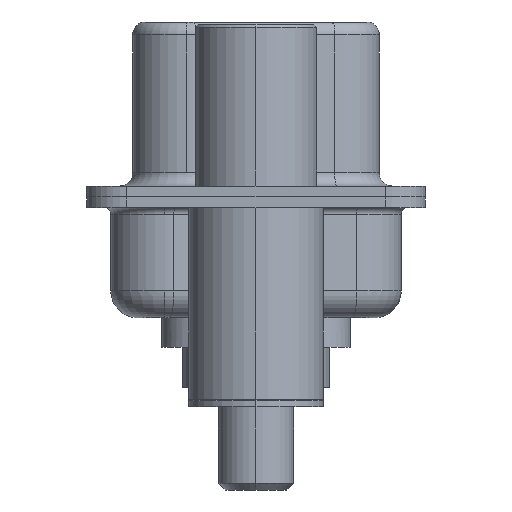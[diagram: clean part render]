
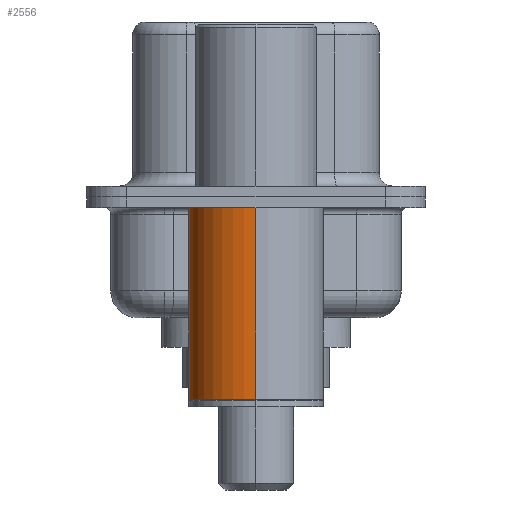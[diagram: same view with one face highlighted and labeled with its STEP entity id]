
A CAD part, left-side view. The second image highlights one B-rep face of the part: STEP entity #2556.
In plain terms, the highlighted cylindrical face has radius 2.5 mm (diameter 5 mm), a partial arc.
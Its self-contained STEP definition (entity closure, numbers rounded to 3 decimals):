
#69 = ORIENTED_EDGE ( 'NONE', *, *, #9008, .F. ) ;
#408 = CARTESIAN_POINT ( 'NONE',  ( -2.5, 0., -0.4 ) ) ;
#678 = DIRECTION ( 'NONE',  ( 0., 0., 1. ) ) ;
#1037 = DIRECTION ( 'NONE',  ( 0., 0., 1. ) ) ;
#2556 = ADVANCED_FACE ( 'NONE', ( #15128 ), #6331, .T. ) ;
#2654 = VERTEX_POINT ( 'NONE', #3700 ) ;
#2798 = CARTESIAN_POINT ( 'NONE',  ( 0., 0., 0.581 ) ) ;
#3330 = CARTESIAN_POINT ( 'NONE',  ( 2.5, 0., 0.581 ) ) ;
#3400 = DIRECTION ( 'NONE',  ( 0., 0., 1. ) ) ;
#3700 = CARTESIAN_POINT ( 'NONE',  ( 2.5, 0., -0.4 ) ) ;
#5219 = CIRCLE ( 'NONE', #7861, 2.5 ) ;
#5476 = ORIENTED_EDGE ( 'NONE', *, *, #16485, .T. ) ;
#6331 = CYLINDRICAL_SURFACE ( 'NONE', #12950, 2.5 ) ;
#6455 = CARTESIAN_POINT ( 'NONE',  ( 0., 0., -7.525 ) ) ;
#7040 = AXIS2_PLACEMENT_3D ( 'NONE', #6455, #18006, #8164 ) ;
#7615 = VERTEX_POINT ( 'NONE', #17468 ) ;
#7847 = LINE ( 'NONE', #3330, #16074 ) ;
#7861 = AXIS2_PLACEMENT_3D ( 'NONE', #10908, #1037, #12555 ) ;
#8020 = EDGE_LOOP ( 'NONE', ( #13777, #5476, #69, #21272 ) ) ;
#8109 = VERTEX_POINT ( 'NONE', #408 ) ;
#8164 = DIRECTION ( 'NONE',  ( 1., 0., 0. ) ) ;
#8531 = VECTOR ( 'NONE', #8851, 1000. ) ;
#8851 = DIRECTION ( 'NONE',  ( 0., 0., 1. ) ) ;
#9008 = EDGE_CURVE ( 'NONE', #2654, #8109, #5219, .T. ) ;
#10472 = VERTEX_POINT ( 'NONE', #19697 ) ;
#10908 = CARTESIAN_POINT ( 'NONE',  ( 0., 0., -0.4 ) ) ;
#11672 = EDGE_CURVE ( 'NONE', #10472, #7615, #12080, .T. ) ;
#12080 = CIRCLE ( 'NONE', #7040, 2.5 ) ;
#12555 = DIRECTION ( 'NONE',  ( 1., 0., 0. ) ) ;
#12835 = LINE ( 'NONE', #15351, #8531 ) ;
#12950 = AXIS2_PLACEMENT_3D ( 'NONE', #2798, #678, #20352 ) ;
#13777 = ORIENTED_EDGE ( 'NONE', *, *, #11672, .T. ) ;
#15128 = FACE_OUTER_BOUND ( 'NONE', #8020, .T. ) ;
#15351 = CARTESIAN_POINT ( 'NONE',  ( -2.5, 0., 0.581 ) ) ;
#16074 = VECTOR ( 'NONE', #3400, 1000. ) ;
#16485 = EDGE_CURVE ( 'NONE', #7615, #8109, #12835, .T. ) ;
#17468 = CARTESIAN_POINT ( 'NONE',  ( -2.5, 0., -7.525 ) ) ;
#18006 = DIRECTION ( 'NONE',  ( 0., 0., 1. ) ) ;
#19697 = CARTESIAN_POINT ( 'NONE',  ( 2.5, 0., -7.525 ) ) ;
#20352 = DIRECTION ( 'NONE',  ( 1., 0., 0. ) ) ;
#21218 = EDGE_CURVE ( 'NONE', #10472, #2654, #7847, .T. ) ;
#21272 = ORIENTED_EDGE ( 'NONE', *, *, #21218, .F. ) ;
